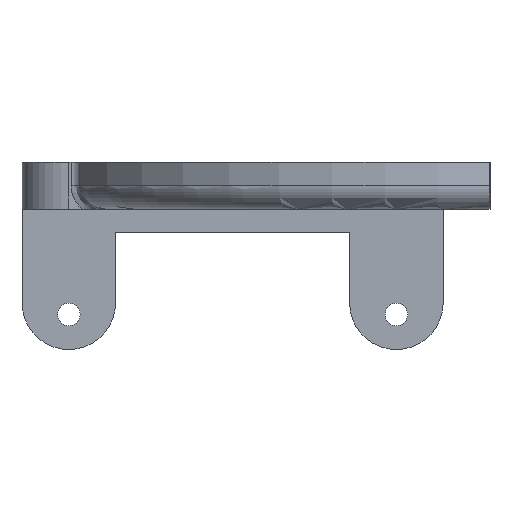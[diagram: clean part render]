
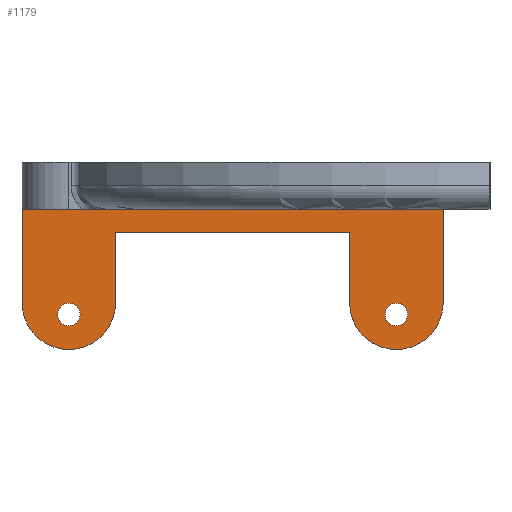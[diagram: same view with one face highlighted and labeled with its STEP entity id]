
A CAD part, left-side view. The second image highlights one B-rep face of the part: STEP entity #1179.
In plain terms, the highlighted planar face has unit normal (-1, 0, 0).
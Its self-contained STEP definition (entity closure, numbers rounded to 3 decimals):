
#10 = VECTOR ( 'NONE', #1907, 1000. ) ;
#15 = VERTEX_POINT ( 'NONE', #1892 ) ;
#17 = AXIS2_PLACEMENT_3D ( 'NONE', #1731, #632, #1926 ) ;
#32 = LINE ( 'NONE', #620, #10 ) ;
#39 = ORIENTED_EDGE ( 'NONE', *, *, #1442, .T. ) ;
#79 = ORIENTED_EDGE ( 'NONE', *, *, #1609, .F. ) ;
#94 = LINE ( 'NONE', #1701, #158 ) ;
#124 = CIRCLE ( 'NONE', #448, 5. ) ;
#128 = AXIS2_PLACEMENT_3D ( 'NONE', #2113, #1024, #2268 ) ;
#150 = CARTESIAN_POINT ( 'NONE',  ( 0., -15., 3.75 ) ) ;
#153 = DIRECTION ( 'NONE',  ( 0., 0., -1. ) ) ;
#157 = DIRECTION ( 'NONE',  ( 0., 0., 1. ) ) ;
#158 = VECTOR ( 'NONE', #1897, 1000. ) ;
#190 = VERTEX_POINT ( 'NONE', #2057 ) ;
#191 = VERTEX_POINT ( 'NONE', #1139 ) ;
#209 = CIRCLE ( 'NONE', #211, 5. ) ;
#211 = AXIS2_PLACEMENT_3D ( 'NONE', #2051, #960, #2216 ) ;
#225 = CARTESIAN_POINT ( 'NONE',  ( 0., -10., -11.25 ) ) ;
#240 = CARTESIAN_POINT ( 'NONE',  ( 0., 30., 3.75 ) ) ;
#252 = CARTESIAN_POINT ( 'NONE',  ( 0., 25., -6.25 ) ) ;
#257 = FACE_BOUND ( 'NONE', #695, .T. ) ;
#259 = CARTESIAN_POINT ( 'NONE',  ( 0., -10., -6.3 ) ) ;
#261 = CIRCLE ( 'NONE', #2262, 1.2 ) ;
#297 = VECTOR ( 'NONE', #1869, 1000. ) ;
#322 = LINE ( 'NONE', #1742, #1201 ) ;
#344 = AXIS2_PLACEMENT_3D ( 'NONE', #1435, #370, #1630 ) ;
#361 = AXIS2_PLACEMENT_3D ( 'NONE', #1571, #1757, #659 ) ;
#370 = DIRECTION ( 'NONE',  ( -1., 0., 0. ) ) ;
#388 = CIRCLE ( 'NONE', #2055, 1.2 ) ;
#393 = ORIENTED_EDGE ( 'NONE', *, *, #1518, .F. ) ;
#415 = DIRECTION ( 'NONE',  ( 0., 0., 1. ) ) ;
#426 = CARTESIAN_POINT ( 'NONE',  ( 0., 25., -11.25 ) ) ;
#448 = AXIS2_PLACEMENT_3D ( 'NONE', #252, #1496, #415 ) ;
#451 = DIRECTION ( 'NONE',  ( -1., 0., 0. ) ) ;
#480 = CIRCLE ( 'NONE', #17, 1.2 ) ;
#488 = PLANE ( 'NONE',  #361 ) ;
#537 = VERTEX_POINT ( 'NONE', #1917 ) ;
#620 = CARTESIAN_POINT ( 'NONE',  ( 0., 20., 1.25 ) ) ;
#632 = DIRECTION ( 'NONE',  ( -1., 0., 0. ) ) ;
#659 = DIRECTION ( 'NONE',  ( 0., 0., 1. ) ) ;
#661 = FACE_BOUND ( 'NONE', #1278, .T. ) ;
#664 = LINE ( 'NONE', #1952, #2053 ) ;
#695 = EDGE_LOOP ( 'NONE', ( #1856, #2037 ) ) ;
#699 = CARTESIAN_POINT ( 'NONE',  ( 0., 25., -8.7 ) ) ;
#702 = CARTESIAN_POINT ( 'NONE',  ( 0., -15., -6.25 ) ) ;
#708 = CARTESIAN_POINT ( 'NONE',  ( 0., 30., -6.25 ) ) ;
#811 = CARTESIAN_POINT ( 'NONE',  ( 0., -10., -8.7 ) ) ;
#822 = DIRECTION ( 'NONE',  ( -1., 0., 0. ) ) ;
#824 = DIRECTION ( 'NONE',  ( 0., 1., 0. ) ) ;
#834 = CARTESIAN_POINT ( 'NONE',  ( 0., -10., -7.5 ) ) ;
#900 = VERTEX_POINT ( 'NONE', #708 ) ;
#904 = VERTEX_POINT ( 'NONE', #702 ) ;
#960 = DIRECTION ( 'NONE',  ( -1., 0., 0. ) ) ;
#967 = EDGE_CURVE ( 'NONE', #537, #190, #1391, .T. ) ;
#970 = CIRCLE ( 'NONE', #128, 5. ) ;
#986 = VERTEX_POINT ( 'NONE', #240 ) ;
#1007 = ORIENTED_EDGE ( 'NONE', *, *, #1438, .F. ) ;
#1022 = DIRECTION ( 'NONE',  ( 0., 0., -1. ) ) ;
#1024 = DIRECTION ( 'NONE',  ( -1., 0., 0. ) ) ;
#1031 = ORIENTED_EDGE ( 'NONE', *, *, #1214, .T. ) ;
#1043 = ORIENTED_EDGE ( 'NONE', *, *, #1136, .F. ) ;
#1067 = EDGE_LOOP ( 'NONE', ( #2149, #2197, #1261, #1043, #39, #2120, #1007, #393, #2166, #1031, #1591 ) ) ;
#1090 = EDGE_CURVE ( 'NONE', #1557, #537, #124, .T. ) ;
#1108 = VERTEX_POINT ( 'NONE', #259 ) ;
#1136 = EDGE_CURVE ( 'NONE', #191, #1489, #94, .T. ) ;
#1139 = CARTESIAN_POINT ( 'NONE',  ( 0., -5., -6.25 ) ) ;
#1175 = VERTEX_POINT ( 'NONE', #150 ) ;
#1179 = ADVANCED_FACE ( 'NONE', ( #2004, #257, #661 ), #488, .T. ) ;
#1186 = VECTOR ( 'NONE', #2161, 1000. ) ;
#1201 = VECTOR ( 'NONE', #824, 1000. ) ;
#1214 = EDGE_CURVE ( 'NONE', #900, #1557, #2255, .T. ) ;
#1224 = CARTESIAN_POINT ( 'NONE',  ( 0., -5., 1.25 ) ) ;
#1261 = ORIENTED_EDGE ( 'NONE', *, *, #1361, .F. ) ;
#1265 = VERTEX_POINT ( 'NONE', #225 ) ;
#1278 = EDGE_LOOP ( 'NONE', ( #79, #1280 ) ) ;
#1280 = ORIENTED_EDGE ( 'NONE', *, *, #1766, .F. ) ;
#1348 = EDGE_CURVE ( 'NONE', #1265, #904, #209, .T. ) ;
#1361 = EDGE_CURVE ( 'NONE', #1489, #1822, #32, .T. ) ;
#1377 = CARTESIAN_POINT ( 'NONE',  ( 0., -15., -3.75 ) ) ;
#1391 = LINE ( 'NONE', #1849, #1186 ) ;
#1399 = LINE ( 'NONE', #1377, #1903 ) ;
#1403 = VERTEX_POINT ( 'NONE', #811 ) ;
#1435 = CARTESIAN_POINT ( 'NONE',  ( 0., 25., -6.25 ) ) ;
#1438 = EDGE_CURVE ( 'NONE', #1175, #904, #1399, .T. ) ;
#1442 = EDGE_CURVE ( 'NONE', #191, #1265, #970, .T. ) ;
#1489 = VERTEX_POINT ( 'NONE', #1224 ) ;
#1496 = DIRECTION ( 'NONE',  ( -1., 0., 0. ) ) ;
#1518 = EDGE_CURVE ( 'NONE', #986, #1175, #1721, .T. ) ;
#1533 = CARTESIAN_POINT ( 'NONE',  ( 0., 25., -7.5 ) ) ;
#1557 = VERTEX_POINT ( 'NONE', #426 ) ;
#1559 = CARTESIAN_POINT ( 'NONE',  ( 0., 12.5, 1.25 ) ) ;
#1571 = CARTESIAN_POINT ( 'NONE',  ( 0., 0., 0. ) ) ;
#1591 = ORIENTED_EDGE ( 'NONE', *, *, #1090, .T. ) ;
#1609 = EDGE_CURVE ( 'NONE', #15, #1943, #480, .T. ) ;
#1630 = DIRECTION ( 'NONE',  ( 0., 0., 1. ) ) ;
#1635 = EDGE_CURVE ( 'NONE', #1822, #190, #322, .T. ) ;
#1647 = EDGE_CURVE ( 'NONE', #1108, #1403, #261, .T. ) ;
#1665 = EDGE_CURVE ( 'NONE', #900, #986, #664, .T. ) ;
#1701 = CARTESIAN_POINT ( 'NONE',  ( 0., -5., -11.25 ) ) ;
#1715 = DIRECTION ( 'NONE',  ( 0., 0., 1. ) ) ;
#1721 = LINE ( 'NONE', #2139, #297 ) ;
#1731 = CARTESIAN_POINT ( 'NONE',  ( 0., 25., -7.5 ) ) ;
#1742 = CARTESIAN_POINT ( 'NONE',  ( 0., 20., 1.25 ) ) ;
#1757 = DIRECTION ( 'NONE',  ( -1., 0., 0. ) ) ;
#1766 = EDGE_CURVE ( 'NONE', #1943, #15, #388, .T. ) ;
#1817 = EDGE_CURVE ( 'NONE', #1403, #1108, #2084, .T. ) ;
#1822 = VERTEX_POINT ( 'NONE', #1559 ) ;
#1849 = CARTESIAN_POINT ( 'NONE',  ( 0., 20., -11.25 ) ) ;
#1856 = ORIENTED_EDGE ( 'NONE', *, *, #1647, .F. ) ;
#1869 = DIRECTION ( 'NONE',  ( 0., -1., 0. ) ) ;
#1892 = CARTESIAN_POINT ( 'NONE',  ( 0., 25., -6.3 ) ) ;
#1897 = DIRECTION ( 'NONE',  ( 0., 0., 1. ) ) ;
#1903 = VECTOR ( 'NONE', #153, 1000. ) ;
#1907 = DIRECTION ( 'NONE',  ( 0., 1., 0. ) ) ;
#1917 = CARTESIAN_POINT ( 'NONE',  ( 0., 20., -6.25 ) ) ;
#1926 = DIRECTION ( 'NONE',  ( 0., 0., 1. ) ) ;
#1939 = CARTESIAN_POINT ( 'NONE',  ( 0., -10., -7.5 ) ) ;
#1943 = VERTEX_POINT ( 'NONE', #699 ) ;
#1952 = CARTESIAN_POINT ( 'NONE',  ( 0., 30., -3.75 ) ) ;
#1987 = AXIS2_PLACEMENT_3D ( 'NONE', #1939, #822, #2100 ) ;
#2004 = FACE_OUTER_BOUND ( 'NONE', #1067, .T. ) ;
#2037 = ORIENTED_EDGE ( 'NONE', *, *, #1817, .F. ) ;
#2051 = CARTESIAN_POINT ( 'NONE',  ( 0., -10., -6.25 ) ) ;
#2053 = VECTOR ( 'NONE', #157, 1000. ) ;
#2055 = AXIS2_PLACEMENT_3D ( 'NONE', #1533, #451, #1715 ) ;
#2057 = CARTESIAN_POINT ( 'NONE',  ( 0., 20., 1.25 ) ) ;
#2084 = CIRCLE ( 'NONE', #1987, 1.2 ) ;
#2100 = DIRECTION ( 'NONE',  ( 0., 0., -1. ) ) ;
#2110 = DIRECTION ( 'NONE',  ( -1., 0., 0. ) ) ;
#2113 = CARTESIAN_POINT ( 'NONE',  ( 0., -10., -6.25 ) ) ;
#2120 = ORIENTED_EDGE ( 'NONE', *, *, #1348, .T. ) ;
#2139 = CARTESIAN_POINT ( 'NONE',  ( 0., 30., 3.75 ) ) ;
#2149 = ORIENTED_EDGE ( 'NONE', *, *, #967, .T. ) ;
#2161 = DIRECTION ( 'NONE',  ( 0., 0., 1. ) ) ;
#2166 = ORIENTED_EDGE ( 'NONE', *, *, #1665, .F. ) ;
#2197 = ORIENTED_EDGE ( 'NONE', *, *, #1635, .F. ) ;
#2216 = DIRECTION ( 'NONE',  ( 0., 0., 1. ) ) ;
#2255 = CIRCLE ( 'NONE', #344, 5. ) ;
#2262 = AXIS2_PLACEMENT_3D ( 'NONE', #834, #2110, #1022 ) ;
#2268 = DIRECTION ( 'NONE',  ( 0., 0., 1. ) ) ;
